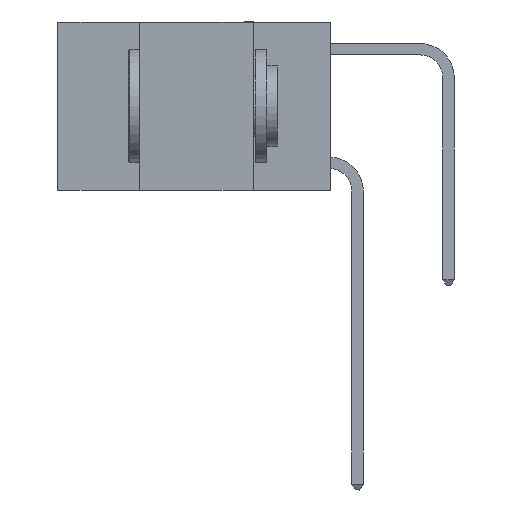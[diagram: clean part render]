
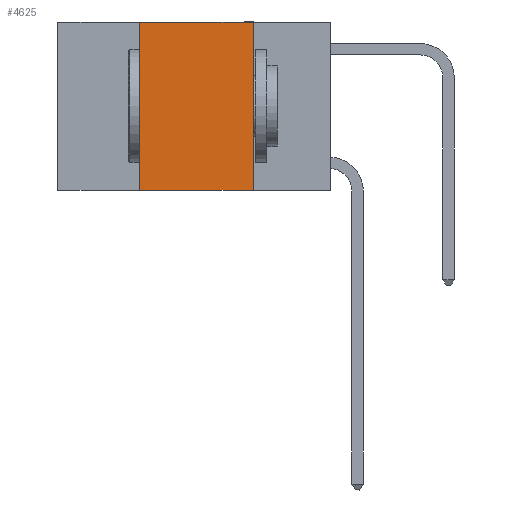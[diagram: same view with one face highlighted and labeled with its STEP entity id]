
A CAD part, left-side view. The second image highlights one B-rep face of the part: STEP entity #4625.
In plain terms, the highlighted planar face has unit normal (-1, 0, 0).
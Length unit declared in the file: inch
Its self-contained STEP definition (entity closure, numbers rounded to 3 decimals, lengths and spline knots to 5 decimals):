
#401 = CARTESIAN_POINT ( 'NONE',  ( 0., 0.17, -0.37 ) ) ;
#2080 = CARTESIAN_POINT ( 'NONE',  ( 0., 0.6, 0. ) ) ;
#3091 = DIRECTION ( 'NONE',  ( 0., -1., 0. ) ) ;
#3973 = EDGE_CURVE ( 'NONE', #29018, #4481, #5470, .T. ) ;
#4481 = VERTEX_POINT ( 'NONE', #12216 ) ;
#4625 = ADVANCED_FACE ( 'NONE', ( #19935 ), #6264, .F. ) ;
#5252 = ORIENTED_EDGE ( 'NONE', *, *, #16185, .T. ) ;
#5470 = LINE ( 'NONE', #7414, #8637 ) ;
#5724 = VERTEX_POINT ( 'NONE', #15688 ) ;
#6264 = PLANE ( 'NONE',  #23660 ) ;
#6780 = LINE ( 'NONE', #26861, #27069 ) ;
#6829 = DIRECTION ( 'NONE',  ( 0., -1., 0. ) ) ;
#6980 = CARTESIAN_POINT ( 'NONE',  ( 0., 0.6, -0.37 ) ) ;
#7414 = CARTESIAN_POINT ( 'NONE',  ( 0., 0.42, 0. ) ) ;
#8449 = EDGE_CURVE ( 'NONE', #4481, #5724, #16916, .T. ) ;
#8519 = DIRECTION ( 'NONE',  ( 1., 0., 0. ) ) ;
#8637 = VECTOR ( 'NONE', #23578, 39.37008 ) ;
#8711 = ORIENTED_EDGE ( 'NONE', *, *, #3973, .F. ) ;
#9571 = VECTOR ( 'NONE', #6829, 39.37008 ) ;
#10357 = CARTESIAN_POINT ( 'NONE',  ( 0., 0.42, -0.37 ) ) ;
#11256 = ORIENTED_EDGE ( 'NONE', *, *, #8449, .F. ) ;
#12216 = CARTESIAN_POINT ( 'NONE',  ( 0., 0.42, 0. ) ) ;
#13311 = DIRECTION ( 'NONE',  ( 0., 0., -1. ) ) ;
#15688 = CARTESIAN_POINT ( 'NONE',  ( 0., 0.17, 0. ) ) ;
#16185 = EDGE_CURVE ( 'NONE', #29018, #25759, #24962, .T. ) ;
#16916 = LINE ( 'NONE', #28061, #24016 ) ;
#17733 = EDGE_LOOP ( 'NONE', ( #23403, #11256, #8711, #5252 ) ) ;
#17855 = DIRECTION ( 'NONE',  ( 0., 0., -1. ) ) ;
#19935 = FACE_OUTER_BOUND ( 'NONE', #17733, .T. ) ;
#23403 = ORIENTED_EDGE ( 'NONE', *, *, #23522, .F. ) ;
#23522 = EDGE_CURVE ( 'NONE', #5724, #25759, #6780, .T. ) ;
#23578 = DIRECTION ( 'NONE',  ( 0., 0., 1. ) ) ;
#23660 = AXIS2_PLACEMENT_3D ( 'NONE', #2080, #8519, #17855 ) ;
#24016 = VECTOR ( 'NONE', #3091, 39.37008 ) ;
#24962 = LINE ( 'NONE', #6980, #9571 ) ;
#25759 = VERTEX_POINT ( 'NONE', #401 ) ;
#26861 = CARTESIAN_POINT ( 'NONE',  ( 0., 0.17, 0. ) ) ;
#27069 = VECTOR ( 'NONE', #13311, 39.37008 ) ;
#28061 = CARTESIAN_POINT ( 'NONE',  ( 0., 0.6, 0. ) ) ;
#29018 = VERTEX_POINT ( 'NONE', #10357 ) ;
